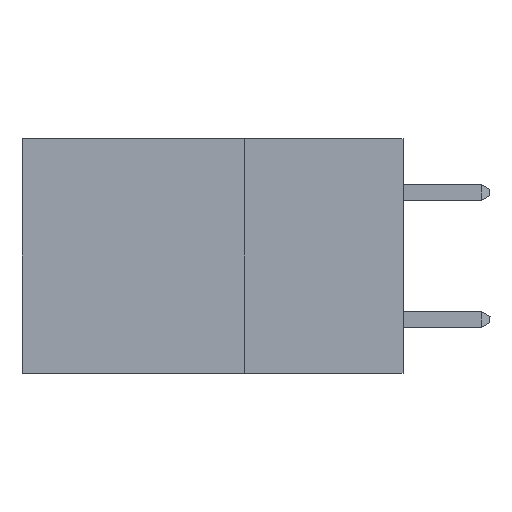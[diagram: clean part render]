
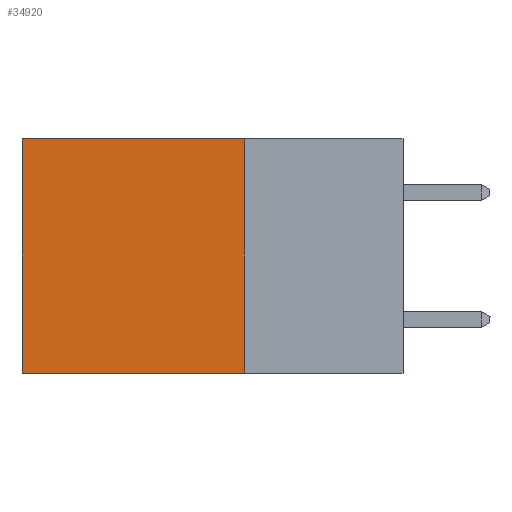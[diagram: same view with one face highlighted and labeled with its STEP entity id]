
A CAD part, left-side view. The second image highlights one B-rep face of the part: STEP entity #34920.
In plain terms, the highlighted planar face has unit normal (-1, 0, 0).
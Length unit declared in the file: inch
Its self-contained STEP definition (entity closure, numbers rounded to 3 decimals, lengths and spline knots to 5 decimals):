
#398 = AXIS2_PLACEMENT_3D ( 'NONE', #26259, #1454, #26727 ) ;
#434 = DIRECTION ( 'NONE',  ( 0., 1., 0. ) ) ;
#826 = VECTOR ( 'NONE', #4801, 39.37008 ) ;
#1089 = LINE ( 'NONE', #43298, #31875 ) ;
#1454 = DIRECTION ( 'NONE',  ( 1., 0., 0. ) ) ;
#3683 = LINE ( 'NONE', #25473, #23643 ) ;
#3730 = CARTESIAN_POINT ( 'NONE',  ( 0.2875, 0.25, 0. ) ) ;
#4801 = DIRECTION ( 'NONE',  ( 0., 0., -1. ) ) ;
#8191 = FACE_OUTER_BOUND ( 'NONE', #29729, .T. ) ;
#9082 = CARTESIAN_POINT ( 'NONE',  ( 0.2875, 0.25, -0.37 ) ) ;
#9098 = PLANE ( 'NONE',  #398 ) ;
#12339 = ORIENTED_EDGE ( 'NONE', *, *, #42373, .F. ) ;
#15248 = EDGE_CURVE ( 'NONE', #25503, #37703, #3683, .T. ) ;
#15539 = CARTESIAN_POINT ( 'NONE',  ( 0.2875, 0.6, -0.37 ) ) ;
#15608 = CARTESIAN_POINT ( 'NONE',  ( 0.2875, 0.6, 0. ) ) ;
#19210 = ORIENTED_EDGE ( 'NONE', *, *, #45216, .T. ) ;
#20139 = ORIENTED_EDGE ( 'NONE', *, *, #15248, .T. ) ;
#23643 = VECTOR ( 'NONE', #434, 39.37008 ) ;
#25473 = CARTESIAN_POINT ( 'NONE',  ( 0.2875, 0.25, 0. ) ) ;
#25503 = VERTEX_POINT ( 'NONE', #34662 ) ;
#25926 = LINE ( 'NONE', #3730, #43292 ) ;
#26259 = CARTESIAN_POINT ( 'NONE',  ( 0.2875, 0.25, 0. ) ) ;
#26727 = DIRECTION ( 'NONE',  ( 0., 0., -1. ) ) ;
#29167 = CARTESIAN_POINT ( 'NONE',  ( 0.2875, 0.6, 0. ) ) ;
#29622 = LINE ( 'NONE', #29167, #826 ) ;
#29729 = EDGE_LOOP ( 'NONE', ( #19210, #12339, #38606, #20139 ) ) ;
#31875 = VECTOR ( 'NONE', #35877, 39.37008 ) ;
#32358 = VERTEX_POINT ( 'NONE', #15539 ) ;
#33951 = EDGE_CURVE ( 'NONE', #25503, #41697, #25926, .T. ) ;
#34662 = CARTESIAN_POINT ( 'NONE',  ( 0.2875, 0.25, 0. ) ) ;
#34920 = ADVANCED_FACE ( 'NONE', ( #8191 ), #9098, .F. ) ;
#35877 = DIRECTION ( 'NONE',  ( 0., 1., 0. ) ) ;
#37703 = VERTEX_POINT ( 'NONE', #15608 ) ;
#38606 = ORIENTED_EDGE ( 'NONE', *, *, #33951, .F. ) ;
#39841 = DIRECTION ( 'NONE',  ( 0., 0., -1. ) ) ;
#41697 = VERTEX_POINT ( 'NONE', #9082 ) ;
#42373 = EDGE_CURVE ( 'NONE', #41697, #32358, #1089, .T. ) ;
#43292 = VECTOR ( 'NONE', #39841, 39.37008 ) ;
#43298 = CARTESIAN_POINT ( 'NONE',  ( 0.2875, 0.25, -0.37 ) ) ;
#45216 = EDGE_CURVE ( 'NONE', #37703, #32358, #29622, .T. ) ;
